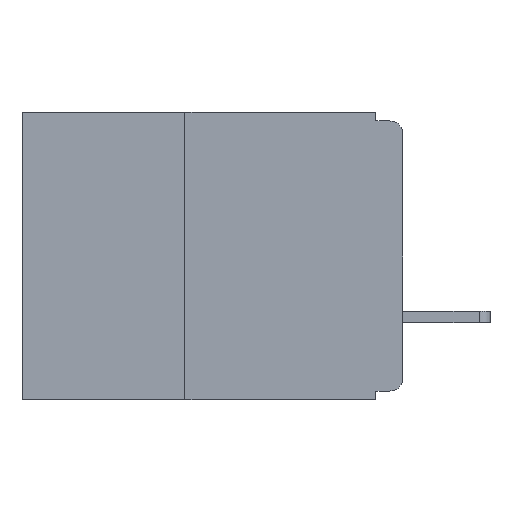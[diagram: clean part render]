
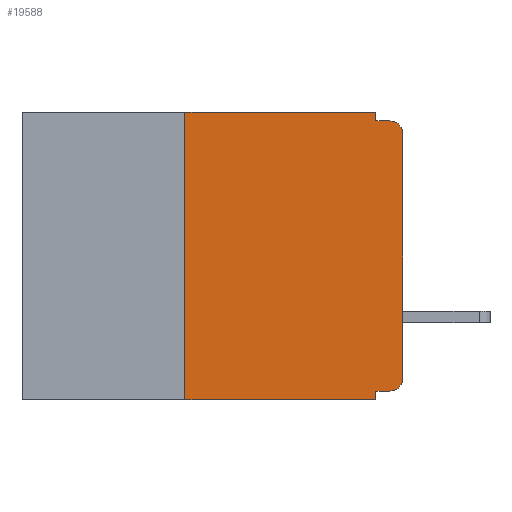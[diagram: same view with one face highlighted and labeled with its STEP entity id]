
A CAD part, left-side view. The second image highlights one B-rep face of the part: STEP entity #19588.
In plain terms, the highlighted planar face has unit normal (-1, 0, 0).
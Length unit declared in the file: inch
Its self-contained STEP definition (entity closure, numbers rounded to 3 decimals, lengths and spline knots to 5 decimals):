
#204 = VERTEX_POINT ( 'NONE', #8438 ) ;
#608 = VERTEX_POINT ( 'NONE', #23265 ) ;
#745 = VECTOR ( 'NONE', #14209, 39.37008 ) ;
#1165 = VECTOR ( 'NONE', #18312, 39.37008 ) ;
#1248 = AXIS2_PLACEMENT_3D ( 'NONE', #8970, #23175, #11037 ) ;
#1475 = CARTESIAN_POINT ( 'NONE',  ( 0., 0., 0. ) ) ;
#1681 = CARTESIAN_POINT ( 'NONE',  ( 0., 0.25, -0.33 ) ) ;
#2078 = ORIENTED_EDGE ( 'NONE', *, *, #23013, .F. ) ;
#2764 = VERTEX_POINT ( 'NONE', #9188 ) ;
#3138 = DIRECTION ( 'NONE',  ( 0., 0., -1. ) ) ;
#3186 = VECTOR ( 'NONE', #25276, 39.37008 ) ;
#3246 = EDGE_CURVE ( 'NONE', #2764, #608, #21991, .T. ) ;
#3344 = ORIENTED_EDGE ( 'NONE', *, *, #8899, .F. ) ;
#3758 = DIRECTION ( 'NONE',  ( 0., 0., 1. ) ) ;
#4073 = CARTESIAN_POINT ( 'NONE',  ( 0., 0.437, 0. ) ) ;
#4154 = EDGE_LOOP ( 'NONE', ( #15392, #6268, #10241, #11511, #16060, #3344, #25697, #2078, #17706, #26027 ) ) ;
#4260 = VERTEX_POINT ( 'NONE', #26441 ) ;
#4695 = CARTESIAN_POINT ( 'NONE',  ( 0., 0., -0.025 ) ) ;
#6268 = ORIENTED_EDGE ( 'NONE', *, *, #8056, .T. ) ;
#6281 = DIRECTION ( 'NONE',  ( 1., 0., 0. ) ) ;
#6870 = VECTOR ( 'NONE', #3138, 39.37008 ) ;
#8056 = EDGE_CURVE ( 'NONE', #16274, #204, #22972, .T. ) ;
#8438 = CARTESIAN_POINT ( 'NONE',  ( 0., 0.015, -0.01 ) ) ;
#8455 = VERTEX_POINT ( 'NONE', #20909 ) ;
#8899 = EDGE_CURVE ( 'NONE', #2764, #25569, #18659, .T. ) ;
#8934 = EDGE_CURVE ( 'NONE', #25185, #204, #11890, .T. ) ;
#8970 = CARTESIAN_POINT ( 'NONE',  ( 0., 0.015, -0.025 ) ) ;
#8986 = CARTESIAN_POINT ( 'NONE',  ( 0., 0.25, 0. ) ) ;
#9116 = CARTESIAN_POINT ( 'NONE',  ( 0., 0., -0.32 ) ) ;
#9188 = CARTESIAN_POINT ( 'NONE',  ( 0., 0.25, -0.33 ) ) ;
#10241 = ORIENTED_EDGE ( 'NONE', *, *, #8934, .F. ) ;
#10430 = CARTESIAN_POINT ( 'NONE',  ( 0., 0.437, 0. ) ) ;
#10733 = DIRECTION ( 'NONE',  ( -1., 0., 0. ) ) ;
#11037 = DIRECTION ( 'NONE',  ( 0., 0., -1. ) ) ;
#11195 = VECTOR ( 'NONE', #22429, 39.37008 ) ;
#11511 = ORIENTED_EDGE ( 'NONE', *, *, #19880, .F. ) ;
#11890 = LINE ( 'NONE', #18405, #745 ) ;
#12300 = LINE ( 'NONE', #20211, #1165 ) ;
#12957 = CARTESIAN_POINT ( 'NONE',  ( 0., 0.031, 0. ) ) ;
#13821 = CIRCLE ( 'NONE', #18621, 0.015 ) ;
#14067 = FACE_OUTER_BOUND ( 'NONE', #4154, .T. ) ;
#14177 = EDGE_CURVE ( 'NONE', #25569, #26151, #20020, .T. ) ;
#14209 = DIRECTION ( 'NONE',  ( 0., -1., 0. ) ) ;
#15015 = EDGE_CURVE ( 'NONE', #8455, #23764, #24943, .T. ) ;
#15392 = ORIENTED_EDGE ( 'NONE', *, *, #25196, .T. ) ;
#15644 = CARTESIAN_POINT ( 'NONE',  ( 0., 0.031, 0. ) ) ;
#15723 = LINE ( 'NONE', #1475, #25674 ) ;
#16060 = ORIENTED_EDGE ( 'NONE', *, *, #14177, .F. ) ;
#16274 = VERTEX_POINT ( 'NONE', #4695 ) ;
#17240 = LINE ( 'NONE', #15644, #6870 ) ;
#17706 = ORIENTED_EDGE ( 'NONE', *, *, #15015, .F. ) ;
#17858 = AXIS2_PLACEMENT_3D ( 'NONE', #4073, #6281, #20659 ) ;
#18312 = DIRECTION ( 'NONE',  ( 0., 0., -1. ) ) ;
#18405 = CARTESIAN_POINT ( 'NONE',  ( 0., 0., -0.01 ) ) ;
#18456 = CARTESIAN_POINT ( 'NONE',  ( 0., 0.031, -0.32 ) ) ;
#18621 = AXIS2_PLACEMENT_3D ( 'NONE', #22879, #10733, #24856 ) ;
#18659 = LINE ( 'NONE', #1681, #19267 ) ;
#18688 = PLANE ( 'NONE',  #17858 ) ;
#19267 = VECTOR ( 'NONE', #3758, 39.37008 ) ;
#19588 = ADVANCED_FACE ( 'NONE', ( #14067 ), #18688, .F. ) ;
#19880 = EDGE_CURVE ( 'NONE', #26151, #25185, #17240, .T. ) ;
#20020 = LINE ( 'NONE', #10430, #24655 ) ;
#20211 = CARTESIAN_POINT ( 'NONE',  ( 0., 0.031, -0.33 ) ) ;
#20659 = DIRECTION ( 'NONE',  ( 0., 0., -1. ) ) ;
#20909 = CARTESIAN_POINT ( 'NONE',  ( 0., 0.015, -0.32 ) ) ;
#21991 = LINE ( 'NONE', #22514, #11195 ) ;
#22070 = DIRECTION ( 'NONE',  ( 0., 0., 1. ) ) ;
#22429 = DIRECTION ( 'NONE',  ( 0., -1., 0. ) ) ;
#22514 = CARTESIAN_POINT ( 'NONE',  ( 0., 0.437, -0.33 ) ) ;
#22585 = DIRECTION ( 'NONE',  ( 0., -1., 0. ) ) ;
#22879 = CARTESIAN_POINT ( 'NONE',  ( 0., 0.015, -0.305 ) ) ;
#22972 = CIRCLE ( 'NONE', #1248, 0.015 ) ;
#23013 = EDGE_CURVE ( 'NONE', #23764, #608, #12300, .T. ) ;
#23175 = DIRECTION ( 'NONE',  ( -1., 0., 0. ) ) ;
#23265 = CARTESIAN_POINT ( 'NONE',  ( 0., 0.031, -0.33 ) ) ;
#23764 = VERTEX_POINT ( 'NONE', #18456 ) ;
#24655 = VECTOR ( 'NONE', #22585, 39.37008 ) ;
#24856 = DIRECTION ( 'NONE',  ( 0., 0., -1. ) ) ;
#24861 = EDGE_CURVE ( 'NONE', #8455, #4260, #13821, .T. ) ;
#24943 = LINE ( 'NONE', #9116, #3186 ) ;
#25185 = VERTEX_POINT ( 'NONE', #25939 ) ;
#25196 = EDGE_CURVE ( 'NONE', #4260, #16274, #15723, .T. ) ;
#25276 = DIRECTION ( 'NONE',  ( 0., 1., 0. ) ) ;
#25569 = VERTEX_POINT ( 'NONE', #8986 ) ;
#25674 = VECTOR ( 'NONE', #22070, 39.37008 ) ;
#25697 = ORIENTED_EDGE ( 'NONE', *, *, #3246, .T. ) ;
#25939 = CARTESIAN_POINT ( 'NONE',  ( 0., 0.031, -0.01 ) ) ;
#26027 = ORIENTED_EDGE ( 'NONE', *, *, #24861, .T. ) ;
#26151 = VERTEX_POINT ( 'NONE', #12957 ) ;
#26441 = CARTESIAN_POINT ( 'NONE',  ( 0., 0., -0.305 ) ) ;
